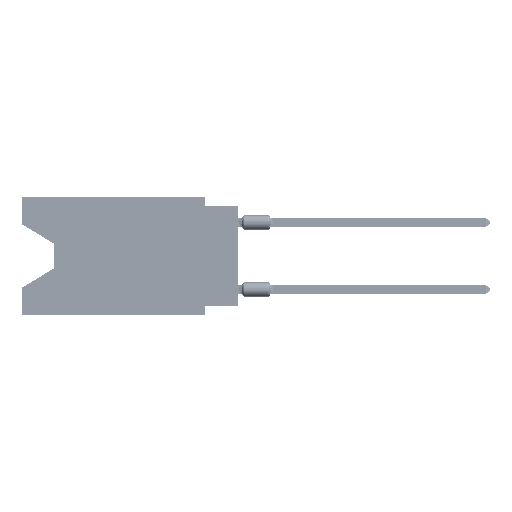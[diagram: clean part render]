
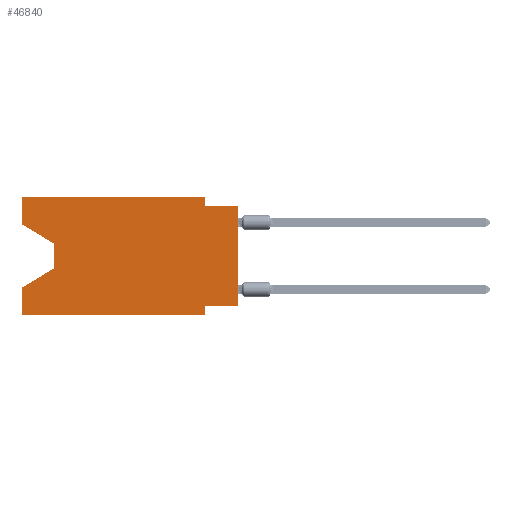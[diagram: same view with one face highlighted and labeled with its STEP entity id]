
A CAD part, left-side view. The second image highlights one B-rep face of the part: STEP entity #46840.
In plain terms, the highlighted planar face has unit normal (-1, 0, 0).
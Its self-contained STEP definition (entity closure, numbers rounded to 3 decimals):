
#197 = LINE ( 'NONE', #57246, #34032 ) ;
#2126 = DIRECTION ( 'NONE',  ( 0., -0.855, -0.519 ) ) ;
#3487 = VECTOR ( 'NONE', #21509, 1000. ) ;
#4787 = AXIS2_PLACEMENT_3D ( 'NONE', #21013, #70376, #15750 ) ;
#5255 = LINE ( 'NONE', #55834, #55082 ) ;
#7643 = LINE ( 'NONE', #69952, #35450 ) ;
#9690 = VERTEX_POINT ( 'NONE', #62696 ) ;
#10165 = ORIENTED_EDGE ( 'NONE', *, *, #60354, .F. ) ;
#11357 = ORIENTED_EDGE ( 'NONE', *, *, #64809, .F. ) ;
#11863 = CARTESIAN_POINT ( 'NONE',  ( 0., 0., -0.635 ) ) ;
#12211 = DIRECTION ( 'NONE',  ( 0., 0., 1. ) ) ;
#13819 = VECTOR ( 'NONE', #12211, 1000. ) ;
#15238 = ORIENTED_EDGE ( 'NONE', *, *, #79641, .F. ) ;
#15454 = CARTESIAN_POINT ( 'NONE',  ( 0., 2.54, 0. ) ) ;
#15750 = DIRECTION ( 'NONE',  ( 0., 0., -1. ) ) ;
#16102 = LINE ( 'NONE', #73116, #42829 ) ;
#17047 = LINE ( 'NONE', #15454, #22951 ) ;
#17352 = VERTEX_POINT ( 'NONE', #77286 ) ;
#17825 = DIRECTION ( 'NONE',  ( 0., 1., 0. ) ) ;
#18737 = CARTESIAN_POINT ( 'NONE',  ( 0., 13.97, -5.385 ) ) ;
#18826 = ORIENTED_EDGE ( 'NONE', *, *, #76141, .F. ) ;
#18838 = DIRECTION ( 'NONE',  ( 0., -1., 0. ) ) ;
#18992 = CARTESIAN_POINT ( 'NONE',  ( 0., 13.97, -3.505 ) ) ;
#19067 = EDGE_CURVE ( 'NONE', #64190, #75029, #32908, .T. ) ;
#20452 = EDGE_CURVE ( 'NONE', #68249, #29469, #197, .T. ) ;
#21013 = CARTESIAN_POINT ( 'NONE',  ( 0., 16.383, 0. ) ) ;
#21509 = DIRECTION ( 'NONE',  ( 0., 0., 1. ) ) ;
#22951 = VECTOR ( 'NONE', #72088, 1000. ) ;
#25627 = VERTEX_POINT ( 'NONE', #33363 ) ;
#25873 = EDGE_CURVE ( 'NONE', #25627, #46312, #44620, .T. ) ;
#25993 = DIRECTION ( 'NONE',  ( 0., 0.855, -0.519 ) ) ;
#26656 = DIRECTION ( 'NONE',  ( 0., -1., 0. ) ) ;
#27174 = LINE ( 'NONE', #34057, #3487 ) ;
#29469 = VERTEX_POINT ( 'NONE', #11863 ) ;
#29771 = LINE ( 'NONE', #52890, #77139 ) ;
#30951 = ORIENTED_EDGE ( 'NONE', *, *, #25873, .T. ) ;
#32908 = LINE ( 'NONE', #57587, #59841 ) ;
#33155 = FACE_OUTER_BOUND ( 'NONE', #41666, .T. ) ;
#33348 = ORIENTED_EDGE ( 'NONE', *, *, #35723, .T. ) ;
#33363 = CARTESIAN_POINT ( 'NONE',  ( 0., 13.97, -5.385 ) ) ;
#33882 = CARTESIAN_POINT ( 'NONE',  ( 0., 2.54, -8.255 ) ) ;
#34032 = VECTOR ( 'NONE', #18838, 1000. ) ;
#34057 = CARTESIAN_POINT ( 'NONE',  ( 0., 16.383, 0. ) ) ;
#35450 = VECTOR ( 'NONE', #26656, 1000. ) ;
#35723 = EDGE_CURVE ( 'NONE', #37313, #41791, #53443, .T. ) ;
#37278 = CARTESIAN_POINT ( 'NONE',  ( 0., 16.383, 0. ) ) ;
#37313 = VERTEX_POINT ( 'NONE', #50259 ) ;
#38117 = CARTESIAN_POINT ( 'NONE',  ( 0., 16.383, -6.852 ) ) ;
#38617 = CARTESIAN_POINT ( 'NONE',  ( 0., 2.54, -0.635 ) ) ;
#40088 = ORIENTED_EDGE ( 'NONE', *, *, #78383, .F. ) ;
#41666 = EDGE_LOOP ( 'NONE', ( #61114, #44928, #30951, #40088, #33348, #43804, #18826, #78404, #70487, #15238, #10165, #11357 ) ) ;
#41791 = VERTEX_POINT ( 'NONE', #64490 ) ;
#42829 = VECTOR ( 'NONE', #59411, 1000. ) ;
#43804 = ORIENTED_EDGE ( 'NONE', *, *, #54885, .F. ) ;
#44294 = EDGE_CURVE ( 'NONE', #68461, #29469, #16102, .T. ) ;
#44620 = LINE ( 'NONE', #18737, #44817 ) ;
#44817 = VECTOR ( 'NONE', #25993, 1000. ) ;
#44928 = ORIENTED_EDGE ( 'NONE', *, *, #78828, .T. ) ;
#46312 = VERTEX_POINT ( 'NONE', #38117 ) ;
#46840 = ADVANCED_FACE ( 'NONE', ( #33155 ), #76447, .F. ) ;
#48404 = DIRECTION ( 'NONE',  ( 0., 0., -1. ) ) ;
#50244 = VERTEX_POINT ( 'NONE', #33882 ) ;
#50259 = CARTESIAN_POINT ( 'NONE',  ( 0., 16.383, -8.89 ) ) ;
#52890 = CARTESIAN_POINT ( 'NONE',  ( 0., 13.97, -3.505 ) ) ;
#53443 = LINE ( 'NONE', #59514, #56138 ) ;
#54885 = EDGE_CURVE ( 'NONE', #50244, #41791, #69246, .T. ) ;
#55082 = VECTOR ( 'NONE', #17825, 1000. ) ;
#55834 = CARTESIAN_POINT ( 'NONE',  ( 0., 0., -8.255 ) ) ;
#56138 = VECTOR ( 'NONE', #70431, 1000. ) ;
#57246 = CARTESIAN_POINT ( 'NONE',  ( 0., 0., -0.635 ) ) ;
#57510 = DIRECTION ( 'NONE',  ( 0., 0., -1. ) ) ;
#57587 = CARTESIAN_POINT ( 'NONE',  ( 0., 16.383, -2.038 ) ) ;
#58330 = VECTOR ( 'NONE', #57510, 1000. ) ;
#59411 = DIRECTION ( 'NONE',  ( 0., 0., 1. ) ) ;
#59514 = CARTESIAN_POINT ( 'NONE',  ( 0., 16.383, -8.89 ) ) ;
#59841 = VECTOR ( 'NONE', #2126, 1000. ) ;
#60354 = EDGE_CURVE ( 'NONE', #9690, #17352, #7643, .T. ) ;
#61114 = ORIENTED_EDGE ( 'NONE', *, *, #19067, .T. ) ;
#61561 = LINE ( 'NONE', #37278, #13819 ) ;
#62696 = CARTESIAN_POINT ( 'NONE',  ( 0., 16.383, 0. ) ) ;
#63576 = CARTESIAN_POINT ( 'NONE',  ( 0., 2.54, -8.89 ) ) ;
#64190 = VERTEX_POINT ( 'NONE', #77081 ) ;
#64490 = CARTESIAN_POINT ( 'NONE',  ( 0., 2.54, -8.89 ) ) ;
#64809 = EDGE_CURVE ( 'NONE', #64190, #9690, #61561, .T. ) ;
#68249 = VERTEX_POINT ( 'NONE', #38617 ) ;
#68461 = VERTEX_POINT ( 'NONE', #72950 ) ;
#69246 = LINE ( 'NONE', #63576, #58330 ) ;
#69952 = CARTESIAN_POINT ( 'NONE',  ( 0., 16.383, 0. ) ) ;
#70376 = DIRECTION ( 'NONE',  ( 1., 0., 0. ) ) ;
#70431 = DIRECTION ( 'NONE',  ( 0., -1., 0. ) ) ;
#70487 = ORIENTED_EDGE ( 'NONE', *, *, #20452, .F. ) ;
#72088 = DIRECTION ( 'NONE',  ( 0., 0., -1. ) ) ;
#72950 = CARTESIAN_POINT ( 'NONE',  ( 0., 0., -8.255 ) ) ;
#73116 = CARTESIAN_POINT ( 'NONE',  ( 0., 0., 0. ) ) ;
#75029 = VERTEX_POINT ( 'NONE', #18992 ) ;
#76141 = EDGE_CURVE ( 'NONE', #68461, #50244, #5255, .T. ) ;
#76447 = PLANE ( 'NONE',  #4787 ) ;
#77081 = CARTESIAN_POINT ( 'NONE',  ( 0., 16.383, -2.038 ) ) ;
#77139 = VECTOR ( 'NONE', #48404, 1000. ) ;
#77286 = CARTESIAN_POINT ( 'NONE',  ( 0., 2.54, 0. ) ) ;
#78383 = EDGE_CURVE ( 'NONE', #37313, #46312, #27174, .T. ) ;
#78404 = ORIENTED_EDGE ( 'NONE', *, *, #44294, .T. ) ;
#78828 = EDGE_CURVE ( 'NONE', #75029, #25627, #29771, .T. ) ;
#79641 = EDGE_CURVE ( 'NONE', #17352, #68249, #17047, .T. ) ;
